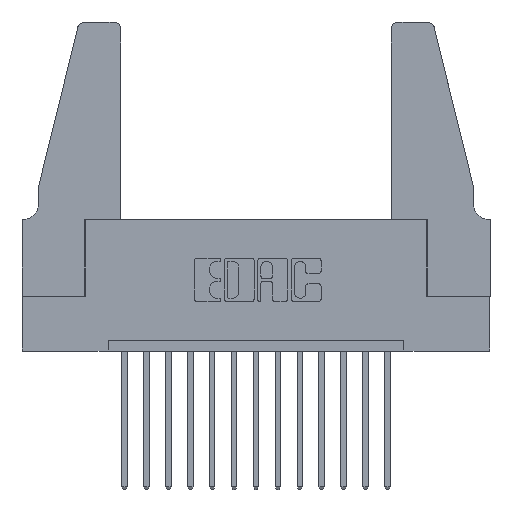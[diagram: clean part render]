
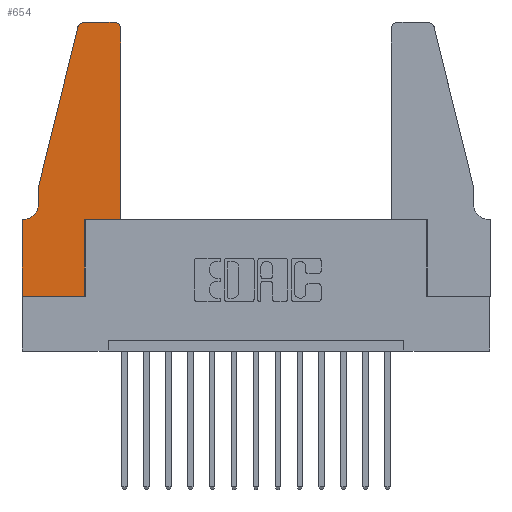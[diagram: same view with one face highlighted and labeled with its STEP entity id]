
A CAD part, top view. The second image highlights one B-rep face of the part: STEP entity #654.
In plain terms, the highlighted planar face has unit normal (0, 0, 1).
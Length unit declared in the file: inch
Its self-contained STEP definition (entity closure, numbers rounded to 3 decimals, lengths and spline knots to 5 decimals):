
#31 = VERTEX_POINT ( 'NONE', #13762 ) ;
#214 = DIRECTION ( 'NONE',  ( 0., 0., 1. ) ) ;
#321 = CARTESIAN_POINT ( 'NONE',  ( 0.4205, 1.22, 0.37 ) ) ;
#433 = VERTEX_POINT ( 'NONE', #6705 ) ;
#475 = ORIENTED_EDGE ( 'NONE', *, *, #5192, .T. ) ;
#549 = DIRECTION ( 'NONE',  ( 0., -1., 0. ) ) ;
#581 = CARTESIAN_POINT ( 'NONE',  ( 0.2865, 0., 0.37 ) ) ;
#592 = ORIENTED_EDGE ( 'NONE', *, *, #10582, .T. ) ;
#654 = ADVANCED_FACE ( 'NONE', ( #6466 ), #2218, .T. ) ;
#815 = CARTESIAN_POINT ( 'NONE',  ( 0.4205, 1.25, 0.37 ) ) ;
#853 = VECTOR ( 'NONE', #6130, 39.37008 ) ;
#868 = LINE ( 'NONE', #3928, #7019 ) ;
#933 = EDGE_CURVE ( 'NONE', #5879, #13470, #7246, .T. ) ;
#1039 = CARTESIAN_POINT ( 'NONE',  ( 0.2865, 0.35, 0.37 ) ) ;
#1505 = EDGE_CURVE ( 'NONE', #14508, #6481, #14689, .T. ) ;
#1869 = DIRECTION ( 'NONE',  ( 0., -1., 0. ) ) ;
#1961 = ORIENTED_EDGE ( 'NONE', *, *, #14277, .T. ) ;
#1966 = AXIS2_PLACEMENT_3D ( 'NONE', #8729, #214, #6400 ) ;
#2218 = PLANE ( 'NONE',  #9219 ) ;
#2283 = VERTEX_POINT ( 'NONE', #5574 ) ;
#2789 = CIRCLE ( 'NONE', #11336, 0.03 ) ;
#2886 = CARTESIAN_POINT ( 'NONE',  ( 0.0755, 0.42, 0.37 ) ) ;
#3024 = CIRCLE ( 'NONE', #10365, 0.07 ) ;
#3303 = DIRECTION ( 'NONE',  ( 0., 0., 1. ) ) ;
#3305 = VECTOR ( 'NONE', #1869, 39.37008 ) ;
#3490 = VECTOR ( 'NONE', #15326, 39.37008 ) ;
#3776 = CARTESIAN_POINT ( 'NONE',  ( 0., 0., 0.37 ) ) ;
#3928 = CARTESIAN_POINT ( 'NONE',  ( 0.0755, 0.35, 0.37 ) ) ;
#4120 = LINE ( 'NONE', #5977, #853 ) ;
#4125 = VECTOR ( 'NONE', #10444, 39.37008 ) ;
#4218 = LINE ( 'NONE', #5334, #11324 ) ;
#4370 = VERTEX_POINT ( 'NONE', #10951 ) ;
#4729 = DIRECTION ( 'NONE',  ( 1., 0., 0. ) ) ;
#4867 = CARTESIAN_POINT ( 'NONE',  ( 0.4505, 0.35, 0.37 ) ) ;
#4937 = EDGE_CURVE ( 'NONE', #433, #14836, #10216, .T. ) ;
#5192 = EDGE_CURVE ( 'NONE', #9087, #433, #4218, .T. ) ;
#5334 = CARTESIAN_POINT ( 'NONE',  ( 0.2605, 1.25, 0.37 ) ) ;
#5574 = CARTESIAN_POINT ( 'NONE',  ( 0.0755, 0.5, 0.37 ) ) ;
#5851 = DIRECTION ( 'NONE',  ( -1., 0., 0. ) ) ;
#5879 = VERTEX_POINT ( 'NONE', #13277 ) ;
#5977 = CARTESIAN_POINT ( 'NONE',  ( 0.0755, 0.5, 0.37 ) ) ;
#6130 = DIRECTION ( 'NONE',  ( -0.239, -0.971, 0. ) ) ;
#6379 = DIRECTION ( 'NONE',  ( -1., 0., 0. ) ) ;
#6388 = ORIENTED_EDGE ( 'NONE', *, *, #4937, .T. ) ;
#6400 = DIRECTION ( 'NONE',  ( 1., 0., 0. ) ) ;
#6458 = ORIENTED_EDGE ( 'NONE', *, *, #1505, .T. ) ;
#6466 = FACE_OUTER_BOUND ( 'NONE', #15801, .T. ) ;
#6481 = VERTEX_POINT ( 'NONE', #12481 ) ;
#6651 = CARTESIAN_POINT ( 'NONE',  ( 0., 0., 0.37 ) ) ;
#6705 = CARTESIAN_POINT ( 'NONE',  ( 0.284, 1.25, 0.37 ) ) ;
#6813 = EDGE_CURVE ( 'NONE', #7684, #14508, #7024, .T. ) ;
#6845 = VECTOR ( 'NONE', #549, 39.37008 ) ;
#6912 = DIRECTION ( 'NONE',  ( 0., 0., -1. ) ) ;
#7019 = VECTOR ( 'NONE', #6379, 39.37008 ) ;
#7024 = LINE ( 'NONE', #1039, #9913 ) ;
#7086 = EDGE_CURVE ( 'NONE', #6481, #31, #15621, .T. ) ;
#7246 = LINE ( 'NONE', #6651, #6845 ) ;
#7684 = VERTEX_POINT ( 'NONE', #581 ) ;
#7764 = CARTESIAN_POINT ( 'NONE',  ( 0.25487, 1.22718, 0.37 ) ) ;
#8601 = DIRECTION ( 'NONE',  ( 0., 1., 0. ) ) ;
#8729 = CARTESIAN_POINT ( 'NONE',  ( 0.284, 1.22, 0.37 ) ) ;
#9087 = VERTEX_POINT ( 'NONE', #815 ) ;
#9104 = ORIENTED_EDGE ( 'NONE', *, *, #13142, .T. ) ;
#9219 = AXIS2_PLACEMENT_3D ( 'NONE', #13163, #3303, #4729 ) ;
#9448 = DIRECTION ( 'NONE',  ( 1., 0., 0. ) ) ;
#9666 = ORIENTED_EDGE ( 'NONE', *, *, #15815, .T. ) ;
#9682 = ORIENTED_EDGE ( 'NONE', *, *, #6813, .T. ) ;
#9759 = DIRECTION ( 'NONE',  ( 0., 0., 1. ) ) ;
#9913 = VECTOR ( 'NONE', #8601, 39.37008 ) ;
#10132 = ORIENTED_EDGE ( 'NONE', *, *, #7086, .T. ) ;
#10216 = CIRCLE ( 'NONE', #1966, 0.03 ) ;
#10302 = CARTESIAN_POINT ( 'NONE',  ( 0.2865, 0.35, 0.37 ) ) ;
#10365 = AXIS2_PLACEMENT_3D ( 'NONE', #15476, #6912, #15642 ) ;
#10444 = DIRECTION ( 'NONE',  ( 0., 1., 0. ) ) ;
#10477 = CARTESIAN_POINT ( 'NONE',  ( 0., 0., 0.37 ) ) ;
#10582 = EDGE_CURVE ( 'NONE', #14468, #4370, #3024, .T. ) ;
#10612 = LINE ( 'NONE', #11551, #3305 ) ;
#10951 = CARTESIAN_POINT ( 'NONE',  ( 0.0055, 0.35, 0.37 ) ) ;
#11324 = VECTOR ( 'NONE', #5851, 39.37008 ) ;
#11336 = AXIS2_PLACEMENT_3D ( 'NONE', #321, #9759, #9448 ) ;
#11429 = VECTOR ( 'NONE', #15377, 39.37008 ) ;
#11494 = ORIENTED_EDGE ( 'NONE', *, *, #933, .T. ) ;
#11551 = CARTESIAN_POINT ( 'NONE',  ( 0.0755, 0.5, 0.37 ) ) ;
#12119 = LINE ( 'NONE', #10477, #3490 ) ;
#12481 = CARTESIAN_POINT ( 'NONE',  ( 0.4505, 0.35, 0.37 ) ) ;
#13142 = EDGE_CURVE ( 'NONE', #31, #9087, #2789, .T. ) ;
#13163 = CARTESIAN_POINT ( 'NONE',  ( 0., 0.35, 0.37 ) ) ;
#13277 = CARTESIAN_POINT ( 'NONE',  ( 0., 0.35, 0.37 ) ) ;
#13368 = ORIENTED_EDGE ( 'NONE', *, *, #13427, .T. ) ;
#13427 = EDGE_CURVE ( 'NONE', #4370, #5879, #868, .T. ) ;
#13470 = VERTEX_POINT ( 'NONE', #3776 ) ;
#13762 = CARTESIAN_POINT ( 'NONE',  ( 0.4505, 1.22, 0.37 ) ) ;
#14277 = EDGE_CURVE ( 'NONE', #14836, #2283, #4120, .T. ) ;
#14468 = VERTEX_POINT ( 'NONE', #2886 ) ;
#14508 = VERTEX_POINT ( 'NONE', #10302 ) ;
#14689 = LINE ( 'NONE', #4867, #11429 ) ;
#14836 = VERTEX_POINT ( 'NONE', #7764 ) ;
#14951 = ORIENTED_EDGE ( 'NONE', *, *, #15272, .T. ) ;
#15272 = EDGE_CURVE ( 'NONE', #2283, #14468, #10612, .T. ) ;
#15305 = CARTESIAN_POINT ( 'NONE',  ( 0.4505, 0.35, 0.37 ) ) ;
#15326 = DIRECTION ( 'NONE',  ( 1., 0., 0. ) ) ;
#15377 = DIRECTION ( 'NONE',  ( 1., 0., 0. ) ) ;
#15476 = CARTESIAN_POINT ( 'NONE',  ( 0.0055, 0.42, 0.37 ) ) ;
#15621 = LINE ( 'NONE', #15305, #4125 ) ;
#15642 = DIRECTION ( 'NONE',  ( -1., 0., 0. ) ) ;
#15801 = EDGE_LOOP ( 'NONE', ( #475, #6388, #1961, #14951, #592, #13368, #11494, #9666, #9682, #6458, #10132, #9104 ) ) ;
#15815 = EDGE_CURVE ( 'NONE', #13470, #7684, #12119, .T. ) ;
